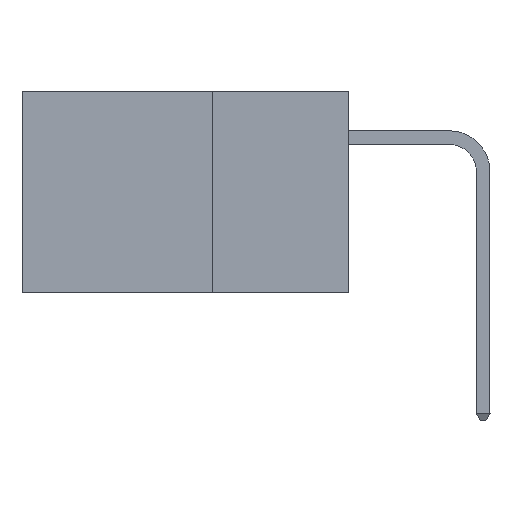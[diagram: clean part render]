
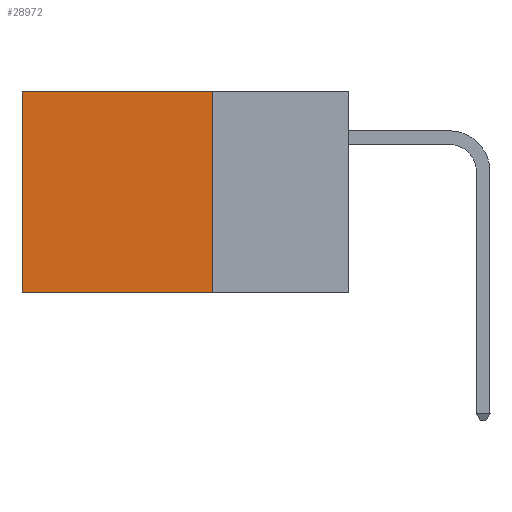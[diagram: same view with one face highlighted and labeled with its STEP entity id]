
A CAD part, left-side view. The second image highlights one B-rep face of the part: STEP entity #28972.
In plain terms, the highlighted planar face has unit normal (-1, 0, 0).
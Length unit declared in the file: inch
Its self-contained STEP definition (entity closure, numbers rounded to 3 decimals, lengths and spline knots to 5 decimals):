
#100 = DIRECTION ( 'NONE',  ( 0., 0., -1. ) ) ;
#726 = PLANE ( 'NONE',  #7469 ) ;
#816 = VECTOR ( 'NONE', #30043, 39.37008 ) ;
#2596 = DIRECTION ( 'NONE',  ( 0., 1., 0. ) ) ;
#5224 = LINE ( 'NONE', #18191, #24843 ) ;
#5832 = VECTOR ( 'NONE', #100, 39.37008 ) ;
#7295 = LINE ( 'NONE', #10294, #5832 ) ;
#7469 = AXIS2_PLACEMENT_3D ( 'NONE', #32817, #23250, #39614 ) ;
#10294 = CARTESIAN_POINT ( 'NONE',  ( 0.2875, 0.25, 0. ) ) ;
#13961 = ORIENTED_EDGE ( 'NONE', *, *, #30447, .T. ) ;
#17489 = CARTESIAN_POINT ( 'NONE',  ( 0.2875, 0.25, 0. ) ) ;
#17649 = EDGE_CURVE ( 'NONE', #37397, #39898, #38116, .T. ) ;
#18191 = CARTESIAN_POINT ( 'NONE',  ( 0.2875, 0.6, 0. ) ) ;
#18426 = EDGE_CURVE ( 'NONE', #35766, #39898, #5224, .T. ) ;
#19944 = CARTESIAN_POINT ( 'NONE',  ( 0.2875, 0.6, 0. ) ) ;
#23250 = DIRECTION ( 'NONE',  ( 1., 0., 0. ) ) ;
#23884 = FACE_OUTER_BOUND ( 'NONE', #29565, .T. ) ;
#24299 = LINE ( 'NONE', #17489, #816 ) ;
#24843 = VECTOR ( 'NONE', #34968, 39.37008 ) ;
#27608 = VECTOR ( 'NONE', #2596, 39.37008 ) ;
#28972 = ADVANCED_FACE ( 'NONE', ( #23884 ), #726, .F. ) ;
#29244 = ORIENTED_EDGE ( 'NONE', *, *, #17649, .F. ) ;
#29565 = EDGE_LOOP ( 'NONE', ( #37293, #29244, #30345, #13961 ) ) ;
#30043 = DIRECTION ( 'NONE',  ( 0., 1., 0. ) ) ;
#30345 = ORIENTED_EDGE ( 'NONE', *, *, #34811, .F. ) ;
#30447 = EDGE_CURVE ( 'NONE', #36900, #35766, #24299, .T. ) ;
#31763 = CARTESIAN_POINT ( 'NONE',  ( 0.2875, 0.25, -0.37 ) ) ;
#32817 = CARTESIAN_POINT ( 'NONE',  ( 0.2875, 0.25, 0. ) ) ;
#34811 = EDGE_CURVE ( 'NONE', #36900, #37397, #7295, .T. ) ;
#34968 = DIRECTION ( 'NONE',  ( 0., 0., -1. ) ) ;
#35766 = VERTEX_POINT ( 'NONE', #19944 ) ;
#36900 = VERTEX_POINT ( 'NONE', #38259 ) ;
#37293 = ORIENTED_EDGE ( 'NONE', *, *, #18426, .T. ) ;
#37397 = VERTEX_POINT ( 'NONE', #31763 ) ;
#38116 = LINE ( 'NONE', #41307, #27608 ) ;
#38259 = CARTESIAN_POINT ( 'NONE',  ( 0.2875, 0.25, 0. ) ) ;
#39614 = DIRECTION ( 'NONE',  ( 0., 0., -1. ) ) ;
#39898 = VERTEX_POINT ( 'NONE', #41606 ) ;
#41307 = CARTESIAN_POINT ( 'NONE',  ( 0.2875, 0.25, -0.37 ) ) ;
#41606 = CARTESIAN_POINT ( 'NONE',  ( 0.2875, 0.6, -0.37 ) ) ;
